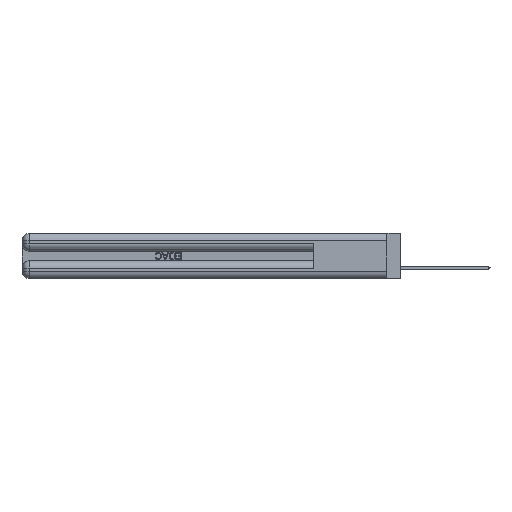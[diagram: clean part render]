
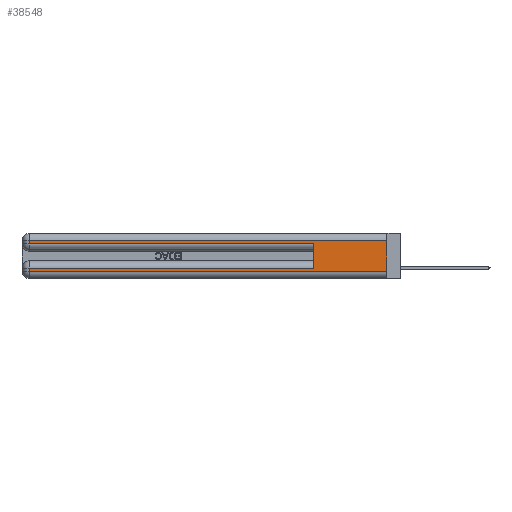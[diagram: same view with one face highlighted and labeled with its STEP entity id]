
A CAD part, left-side view. The second image highlights one B-rep face of the part: STEP entity #38548.
In plain terms, the highlighted planar face has unit normal (-1, 0, 0).
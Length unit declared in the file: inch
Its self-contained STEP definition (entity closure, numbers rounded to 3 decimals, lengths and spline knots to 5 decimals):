
#1452 = EDGE_CURVE ( 'NONE', #31998, #30032, #34247, .T. ) ;
#1763 = VERTEX_POINT ( 'NONE', #37638 ) ;
#2380 = VECTOR ( 'NONE', #14984, 39.37008 ) ;
#4572 = ORIENTED_EDGE ( 'NONE', *, *, #37731, .T. ) ;
#4849 = LINE ( 'NONE', #26260, #25459 ) ;
#7937 = CARTESIAN_POINT ( 'NONE',  ( 0., 2.94, 0.285 ) ) ;
#9112 = ORIENTED_EDGE ( 'NONE', *, *, #33976, .T. ) ;
#9435 = DIRECTION ( 'NONE',  ( 1., 0., 0. ) ) ;
#9469 = ORIENTED_EDGE ( 'NONE', *, *, #28283, .F. ) ;
#9606 = CARTESIAN_POINT ( 'NONE',  ( 0., 0., 0.37 ) ) ;
#9777 = DIRECTION ( 'NONE',  ( 0., 0., -1. ) ) ;
#10707 = CARTESIAN_POINT ( 'NONE',  ( 0., 0.6, 0.285 ) ) ;
#10824 = CARTESIAN_POINT ( 'NONE',  ( 0., 0., 0.37 ) ) ;
#11277 = LINE ( 'NONE', #51225, #41882 ) ;
#11621 = VERTEX_POINT ( 'NONE', #36012 ) ;
#13789 = VERTEX_POINT ( 'NONE', #10707 ) ;
#14984 = DIRECTION ( 'NONE',  ( 0., 0., -1. ) ) ;
#17356 = ORIENTED_EDGE ( 'NONE', *, *, #26059, .T. ) ;
#19057 = VECTOR ( 'NONE', #20969, 39.37008 ) ;
#20508 = CARTESIAN_POINT ( 'NONE',  ( 0., 0., 0.06 ) ) ;
#20969 = DIRECTION ( 'NONE',  ( 0., 1., 0. ) ) ;
#20976 = AXIS2_PLACEMENT_3D ( 'NONE', #9606, #9435, #9777 ) ;
#21898 = FACE_OUTER_BOUND ( 'NONE', #24184, .T. ) ;
#22121 = VERTEX_POINT ( 'NONE', #7937 ) ;
#23044 = CARTESIAN_POINT ( 'NONE',  ( 0., 0., 0.06 ) ) ;
#24184 = EDGE_LOOP ( 'NONE', ( #46743, #37939, #17356, #46376, #9469, #26064, #4572, #9112 ) ) ;
#24207 = LINE ( 'NONE', #20508, #28552 ) ;
#25459 = VECTOR ( 'NONE', #33767, 39.37008 ) ;
#25921 = LINE ( 'NONE', #29588, #43520 ) ;
#26059 = EDGE_CURVE ( 'NONE', #11621, #22121, #50166, .T. ) ;
#26064 = ORIENTED_EDGE ( 'NONE', *, *, #29632, .T. ) ;
#26260 = CARTESIAN_POINT ( 'NONE',  ( 0., 0.6, 0.145 ) ) ;
#27079 = DIRECTION ( 'NONE',  ( 0., 1., 0. ) ) ;
#28283 = EDGE_CURVE ( 'NONE', #1763, #13789, #4849, .T. ) ;
#28552 = VECTOR ( 'NONE', #44370, 39.37008 ) ;
#28618 = CARTESIAN_POINT ( 'NONE',  ( 0., 2.94, 0.37 ) ) ;
#28700 = CARTESIAN_POINT ( 'NONE',  ( 0., 2.94, 0.085 ) ) ;
#29588 = CARTESIAN_POINT ( 'NONE',  ( 0., 0., 0.285 ) ) ;
#29632 = EDGE_CURVE ( 'NONE', #1763, #42189, #42880, .T. ) ;
#30032 = VERTEX_POINT ( 'NONE', #23044 ) ;
#31998 = VERTEX_POINT ( 'NONE', #48762 ) ;
#33363 = PLANE ( 'NONE',  #20976 ) ;
#33767 = DIRECTION ( 'NONE',  ( 0., 0., 1. ) ) ;
#33976 = EDGE_CURVE ( 'NONE', #33994, #30032, #24207, .T. ) ;
#33994 = VERTEX_POINT ( 'NONE', #36448 ) ;
#34247 = LINE ( 'NONE', #10824, #2380 ) ;
#35792 = LINE ( 'NONE', #46907, #45188 ) ;
#36012 = CARTESIAN_POINT ( 'NONE',  ( 0., 2.94, 0.31 ) ) ;
#36055 = EDGE_CURVE ( 'NONE', #22121, #13789, #25921, .T. ) ;
#36448 = CARTESIAN_POINT ( 'NONE',  ( 0., 2.94, 0.06 ) ) ;
#37638 = CARTESIAN_POINT ( 'NONE',  ( 0., 0.6, 0.085 ) ) ;
#37731 = EDGE_CURVE ( 'NONE', #42189, #33994, #35792, .T. ) ;
#37939 = ORIENTED_EDGE ( 'NONE', *, *, #38833, .T. ) ;
#38256 = VECTOR ( 'NONE', #49965, 39.37008 ) ;
#38548 = ADVANCED_FACE ( 'NONE', ( #21898 ), #33363, .F. ) ;
#38833 = EDGE_CURVE ( 'NONE', #31998, #11621, #11277, .T. ) ;
#40606 = CARTESIAN_POINT ( 'NONE',  ( 0., 0., 0.085 ) ) ;
#40939 = DIRECTION ( 'NONE',  ( 0., -1., 0. ) ) ;
#41882 = VECTOR ( 'NONE', #27079, 39.37008 ) ;
#42189 = VERTEX_POINT ( 'NONE', #28700 ) ;
#42880 = LINE ( 'NONE', #40606, #19057 ) ;
#43520 = VECTOR ( 'NONE', #40939, 39.37008 ) ;
#44370 = DIRECTION ( 'NONE',  ( 0., -1., 0. ) ) ;
#45188 = VECTOR ( 'NONE', #50905, 39.37008 ) ;
#46376 = ORIENTED_EDGE ( 'NONE', *, *, #36055, .T. ) ;
#46743 = ORIENTED_EDGE ( 'NONE', *, *, #1452, .F. ) ;
#46907 = CARTESIAN_POINT ( 'NONE',  ( 0., 2.94, 0.37 ) ) ;
#48762 = CARTESIAN_POINT ( 'NONE',  ( 0., 0., 0.31 ) ) ;
#49965 = DIRECTION ( 'NONE',  ( 0., 0., -1. ) ) ;
#50166 = LINE ( 'NONE', #28618, #38256 ) ;
#50905 = DIRECTION ( 'NONE',  ( 0., 0., -1. ) ) ;
#51225 = CARTESIAN_POINT ( 'NONE',  ( 0., 0., 0.31 ) ) ;
